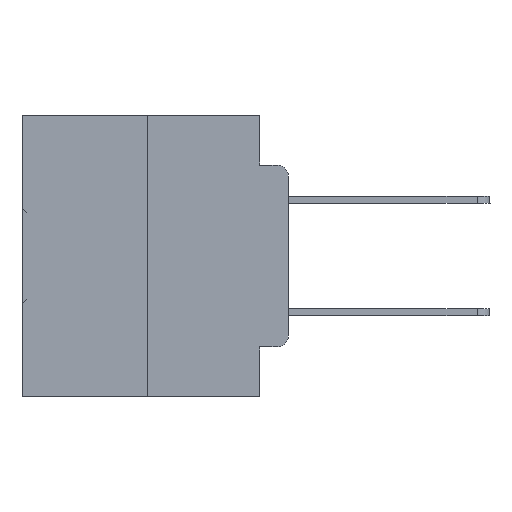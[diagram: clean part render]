
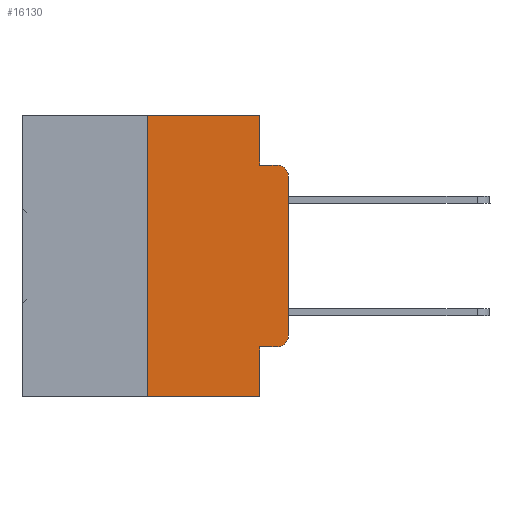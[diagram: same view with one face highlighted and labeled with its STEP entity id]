
A CAD part, left-side view. The second image highlights one B-rep face of the part: STEP entity #16130.
In plain terms, the highlighted planar face has unit normal (-1, 0, 0).
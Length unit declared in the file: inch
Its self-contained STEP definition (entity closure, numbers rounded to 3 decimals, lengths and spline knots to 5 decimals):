
#282 = LINE ( 'NONE', #22808, #12162 ) ;
#1128 = DIRECTION ( 'NONE',  ( 0., 0., -1. ) ) ;
#1442 = CARTESIAN_POINT ( 'NONE',  ( 0., 0., -0.1085 ) ) ;
#1793 = VECTOR ( 'NONE', #27438, 39.37008 ) ;
#3341 = EDGE_LOOP ( 'NONE', ( #11273, #13400, #31266, #29121, #22592, #11254, #31638, #12858, #16184, #35468 ) ) ;
#3423 = DIRECTION ( 'NONE',  ( -1., 0., 0. ) ) ;
#3524 = EDGE_CURVE ( 'NONE', #15613, #5089, #28233, .T. ) ;
#4430 = CARTESIAN_POINT ( 'NONE',  ( 0., 0.051, -0.0885 ) ) ;
#4546 = CARTESIAN_POINT ( 'NONE',  ( 0., 0.02, -0.0885 ) ) ;
#5089 = VERTEX_POINT ( 'NONE', #1442 ) ;
#5261 = EDGE_CURVE ( 'NONE', #5089, #30063, #20253, .T. ) ;
#5690 = LINE ( 'NONE', #22204, #10524 ) ;
#5722 = VERTEX_POINT ( 'NONE', #27810 ) ;
#5810 = VERTEX_POINT ( 'NONE', #14347 ) ;
#6167 = CARTESIAN_POINT ( 'NONE',  ( 0., 0., -0.3915 ) ) ;
#6604 = CARTESIAN_POINT ( 'NONE',  ( 0., 0.051, 0. ) ) ;
#7416 = DIRECTION ( 'NONE',  ( 0., -1., 0. ) ) ;
#7620 = VERTEX_POINT ( 'NONE', #33965 ) ;
#8087 = VECTOR ( 'NONE', #16844, 39.37008 ) ;
#8918 = DIRECTION ( 'NONE',  ( 0., 0., 1. ) ) ;
#8944 = VERTEX_POINT ( 'NONE', #23125 ) ;
#9062 = FACE_OUTER_BOUND ( 'NONE', #3341, .T. ) ;
#10524 = VECTOR ( 'NONE', #33412, 39.37008 ) ;
#11067 = LINE ( 'NONE', #33495, #33510 ) ;
#11078 = DIRECTION ( 'NONE',  ( 0., 0., -1. ) ) ;
#11254 = ORIENTED_EDGE ( 'NONE', *, *, #22138, .F. ) ;
#11273 = ORIENTED_EDGE ( 'NONE', *, *, #3524, .T. ) ;
#12162 = VECTOR ( 'NONE', #28178, 39.37008 ) ;
#12858 = ORIENTED_EDGE ( 'NONE', *, *, #20139, .F. ) ;
#13221 = AXIS2_PLACEMENT_3D ( 'NONE', #17321, #3423, #11078 ) ;
#13400 = ORIENTED_EDGE ( 'NONE', *, *, #5261, .T. ) ;
#13675 = CIRCLE ( 'NONE', #33651, 0.02 ) ;
#14008 = DIRECTION ( 'NONE',  ( 0., 0., -1. ) ) ;
#14347 = CARTESIAN_POINT ( 'NONE',  ( 0., 0.02, -0.4115 ) ) ;
#14722 = VECTOR ( 'NONE', #1128, 39.37008 ) ;
#15194 = EDGE_CURVE ( 'NONE', #7620, #30063, #32351, .T. ) ;
#15613 = VERTEX_POINT ( 'NONE', #6167 ) ;
#15627 = CARTESIAN_POINT ( 'NONE',  ( 0., 0.051, -0.4115 ) ) ;
#16130 = ADVANCED_FACE ( 'NONE', ( #9062 ), #30570, .F. ) ;
#16184 = ORIENTED_EDGE ( 'NONE', *, *, #29771, .T. ) ;
#16514 = DIRECTION ( 'NONE',  ( 0., 0., -1. ) ) ;
#16577 = DIRECTION ( 'NONE',  ( 0., 0., 1. ) ) ;
#16675 = VERTEX_POINT ( 'NONE', #17778 ) ;
#16751 = CARTESIAN_POINT ( 'NONE',  ( 0., 0.473, 0. ) ) ;
#16844 = DIRECTION ( 'NONE',  ( 0., -1., 0. ) ) ;
#17321 = CARTESIAN_POINT ( 'NONE',  ( 0., 0.02, -0.1085 ) ) ;
#17577 = VERTEX_POINT ( 'NONE', #24993 ) ;
#17778 = CARTESIAN_POINT ( 'NONE',  ( 0., 0.25, 0. ) ) ;
#18740 = EDGE_CURVE ( 'NONE', #16675, #21629, #5690, .T. ) ;
#18923 = LINE ( 'NONE', #15627, #1793 ) ;
#20139 = EDGE_CURVE ( 'NONE', #17577, #5722, #34132, .T. ) ;
#20253 = CIRCLE ( 'NONE', #13221, 0.02 ) ;
#21629 = VERTEX_POINT ( 'NONE', #31408 ) ;
#22138 = EDGE_CURVE ( 'NONE', #8944, #16675, #11067, .T. ) ;
#22204 = CARTESIAN_POINT ( 'NONE',  ( 0., 0.473, 0. ) ) ;
#22592 = ORIENTED_EDGE ( 'NONE', *, *, #18740, .F. ) ;
#22808 = CARTESIAN_POINT ( 'NONE',  ( 0., 0.051, 0. ) ) ;
#23125 = CARTESIAN_POINT ( 'NONE',  ( 0., 0.25, -0.5 ) ) ;
#24993 = CARTESIAN_POINT ( 'NONE',  ( 0., 0.051, -0.4115 ) ) ;
#25114 = EDGE_CURVE ( 'NONE', #21629, #7620, #282, .T. ) ;
#25995 = EDGE_CURVE ( 'NONE', #8944, #5722, #31865, .T. ) ;
#26388 = CARTESIAN_POINT ( 'NONE',  ( 0., 0.473, -0.5 ) ) ;
#27047 = VECTOR ( 'NONE', #8918, 39.37008 ) ;
#27438 = DIRECTION ( 'NONE',  ( 0., -1., 0. ) ) ;
#27603 = DIRECTION ( 'NONE',  ( -1., 0., 0. ) ) ;
#27810 = CARTESIAN_POINT ( 'NONE',  ( 0., 0.051, -0.5 ) ) ;
#28018 = DIRECTION ( 'NONE',  ( 1., 0., 0. ) ) ;
#28026 = AXIS2_PLACEMENT_3D ( 'NONE', #16751, #28018, #14008 ) ;
#28178 = DIRECTION ( 'NONE',  ( 0., 0., -1. ) ) ;
#28233 = LINE ( 'NONE', #29287, #27047 ) ;
#29121 = ORIENTED_EDGE ( 'NONE', *, *, #25114, .F. ) ;
#29287 = CARTESIAN_POINT ( 'NONE',  ( 0., 0., 0. ) ) ;
#29771 = EDGE_CURVE ( 'NONE', #17577, #5810, #18923, .T. ) ;
#29791 = CARTESIAN_POINT ( 'NONE',  ( 0., 0.02, -0.3915 ) ) ;
#30063 = VERTEX_POINT ( 'NONE', #4546 ) ;
#30570 = PLANE ( 'NONE',  #28026 ) ;
#31266 = ORIENTED_EDGE ( 'NONE', *, *, #15194, .F. ) ;
#31408 = CARTESIAN_POINT ( 'NONE',  ( 0., 0.051, 0. ) ) ;
#31638 = ORIENTED_EDGE ( 'NONE', *, *, #25995, .T. ) ;
#31865 = LINE ( 'NONE', #26388, #32738 ) ;
#32351 = LINE ( 'NONE', #4430, #8087 ) ;
#32738 = VECTOR ( 'NONE', #7416, 39.37008 ) ;
#33412 = DIRECTION ( 'NONE',  ( 0., -1., 0. ) ) ;
#33495 = CARTESIAN_POINT ( 'NONE',  ( 0., 0.25, 0. ) ) ;
#33510 = VECTOR ( 'NONE', #16577, 39.37008 ) ;
#33651 = AXIS2_PLACEMENT_3D ( 'NONE', #29791, #27603, #16514 ) ;
#33965 = CARTESIAN_POINT ( 'NONE',  ( 0., 0.051, -0.0885 ) ) ;
#34132 = LINE ( 'NONE', #6604, #14722 ) ;
#35468 = ORIENTED_EDGE ( 'NONE', *, *, #35744, .T. ) ;
#35744 = EDGE_CURVE ( 'NONE', #5810, #15613, #13675, .T. ) ;
